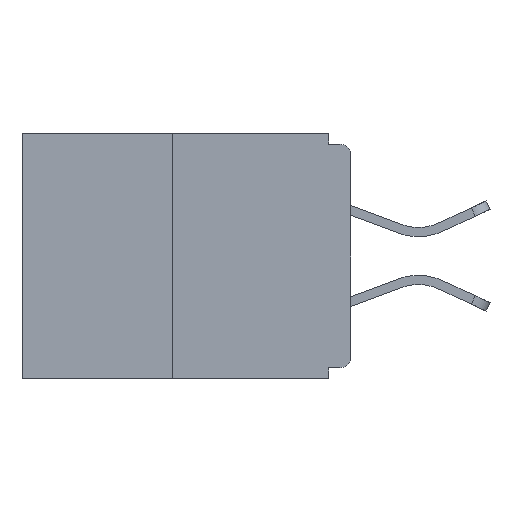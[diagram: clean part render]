
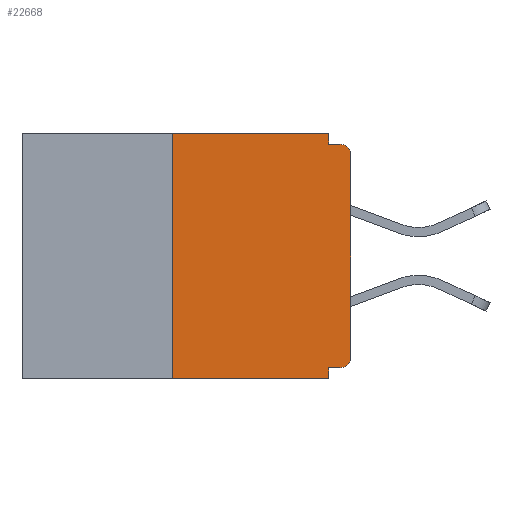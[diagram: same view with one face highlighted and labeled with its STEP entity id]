
A CAD part, left-side view. The second image highlights one B-rep face of the part: STEP entity #22668.
In plain terms, the highlighted planar face has unit normal (-1, 0, 0).
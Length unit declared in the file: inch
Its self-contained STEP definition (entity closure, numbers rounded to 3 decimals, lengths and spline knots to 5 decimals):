
#311 = ORIENTED_EDGE ( 'NONE', *, *, #23160, .F. ) ;
#749 = CARTESIAN_POINT ( 'NONE',  ( 0., 0.46, 0. ) ) ;
#984 = DIRECTION ( 'NONE',  ( -1., 0., 0. ) ) ;
#1036 = VERTEX_POINT ( 'NONE', #2651 ) ;
#1200 = VECTOR ( 'NONE', #20123, 39.37008 ) ;
#1332 = VERTEX_POINT ( 'NONE', #11751 ) ;
#1795 = EDGE_CURVE ( 'NONE', #21712, #1036, #19351, .T. ) ;
#2651 = CARTESIAN_POINT ( 'NONE',  ( 0., 0.015, -0.015 ) ) ;
#2827 = VECTOR ( 'NONE', #16378, 39.37008 ) ;
#3224 = EDGE_LOOP ( 'NONE', ( #311, #25900, #19382, #6486, #30759, #19898, #22731, #23529, #9646, #14262 ) ) ;
#3354 = CARTESIAN_POINT ( 'NONE',  ( 0., 0.25, 0. ) ) ;
#3459 = CARTESIAN_POINT ( 'NONE',  ( 0., 0., 0. ) ) ;
#3608 = CARTESIAN_POINT ( 'NONE',  ( 0., 0.46, -0.343 ) ) ;
#4226 = AXIS2_PLACEMENT_3D ( 'NONE', #27526, #984, #18160 ) ;
#4317 = LINE ( 'NONE', #17866, #1200 ) ;
#6371 = LINE ( 'NONE', #19010, #9063 ) ;
#6486 = ORIENTED_EDGE ( 'NONE', *, *, #20526, .F. ) ;
#7326 = LINE ( 'NONE', #22070, #20362 ) ;
#7821 = VERTEX_POINT ( 'NONE', #9817 ) ;
#8013 = LINE ( 'NONE', #3608, #18004 ) ;
#8146 = DIRECTION ( 'NONE',  ( 1., 0., 0. ) ) ;
#8205 = CARTESIAN_POINT ( 'NONE',  ( 0., 0., -0.328 ) ) ;
#9063 = VECTOR ( 'NONE', #26462, 39.37008 ) ;
#9182 = CARTESIAN_POINT ( 'NONE',  ( 0., 0., -0.313 ) ) ;
#9421 = VERTEX_POINT ( 'NONE', #27793 ) ;
#9646 = ORIENTED_EDGE ( 'NONE', *, *, #12919, .F. ) ;
#9674 = VERTEX_POINT ( 'NONE', #25311 ) ;
#9817 = CARTESIAN_POINT ( 'NONE',  ( 0., 0.015, -0.328 ) ) ;
#10089 = LINE ( 'NONE', #15951, #26540 ) ;
#10485 = LINE ( 'NONE', #3459, #14682 ) ;
#10829 = DIRECTION ( 'NONE',  ( 0., 0., -1. ) ) ;
#11751 = CARTESIAN_POINT ( 'NONE',  ( 0., 0.25, -0.343 ) ) ;
#12376 = AXIS2_PLACEMENT_3D ( 'NONE', #749, #8146, #10829 ) ;
#12567 = VERTEX_POINT ( 'NONE', #3354 ) ;
#12919 = EDGE_CURVE ( 'NONE', #9421, #1036, #7326, .T. ) ;
#14188 = CARTESIAN_POINT ( 'NONE',  ( 0., 0.031, 0. ) ) ;
#14262 = ORIENTED_EDGE ( 'NONE', *, *, #23239, .F. ) ;
#14634 = DIRECTION ( 'NONE',  ( 0., -1., 0. ) ) ;
#14682 = VECTOR ( 'NONE', #22709, 39.37008 ) ;
#15905 = DIRECTION ( 'NONE',  ( 0., -1., 0. ) ) ;
#15951 = CARTESIAN_POINT ( 'NONE',  ( 0., 0.46, 0. ) ) ;
#16243 = CIRCLE ( 'NONE', #28810, 0.015 ) ;
#16259 = VERTEX_POINT ( 'NONE', #31473 ) ;
#16378 = DIRECTION ( 'NONE',  ( 0., 0., -1. ) ) ;
#16776 = EDGE_CURVE ( 'NONE', #7821, #9674, #26425, .T. ) ;
#16782 = CARTESIAN_POINT ( 'NONE',  ( 0., 0., -0.03 ) ) ;
#17866 = CARTESIAN_POINT ( 'NONE',  ( 0., 0.031, -0.343 ) ) ;
#18004 = VECTOR ( 'NONE', #15905, 39.37008 ) ;
#18026 = PLANE ( 'NONE',  #12376 ) ;
#18160 = DIRECTION ( 'NONE',  ( 0., 0., -1. ) ) ;
#19010 = CARTESIAN_POINT ( 'NONE',  ( 0., 0.25, 0. ) ) ;
#19342 = FACE_OUTER_BOUND ( 'NONE', #3224, .T. ) ;
#19351 = CIRCLE ( 'NONE', #4226, 0.015 ) ;
#19382 = ORIENTED_EDGE ( 'NONE', *, *, #25205, .T. ) ;
#19898 = ORIENTED_EDGE ( 'NONE', *, *, #22839, .T. ) ;
#20123 = DIRECTION ( 'NONE',  ( 0., 0., -1. ) ) ;
#20362 = VECTOR ( 'NONE', #14634, 39.37008 ) ;
#20451 = DIRECTION ( 'NONE',  ( 0., 1., 0. ) ) ;
#20526 = EDGE_CURVE ( 'NONE', #9674, #25125, #4317, .T. ) ;
#20714 = VECTOR ( 'NONE', #20451, 39.37008 ) ;
#21712 = VERTEX_POINT ( 'NONE', #16782 ) ;
#22070 = CARTESIAN_POINT ( 'NONE',  ( 0., 0., -0.015 ) ) ;
#22668 = ADVANCED_FACE ( 'NONE', ( #19342 ), #18026, .F. ) ;
#22709 = DIRECTION ( 'NONE',  ( 0., 0., 1. ) ) ;
#22731 = ORIENTED_EDGE ( 'NONE', *, *, #22766, .T. ) ;
#22766 = EDGE_CURVE ( 'NONE', #24740, #21712, #10485, .T. ) ;
#22839 = EDGE_CURVE ( 'NONE', #7821, #24740, #16243, .T. ) ;
#23160 = EDGE_CURVE ( 'NONE', #12567, #16259, #10089, .T. ) ;
#23239 = EDGE_CURVE ( 'NONE', #16259, #9421, #31163, .T. ) ;
#23529 = ORIENTED_EDGE ( 'NONE', *, *, #1795, .T. ) ;
#24740 = VERTEX_POINT ( 'NONE', #9182 ) ;
#25125 = VERTEX_POINT ( 'NONE', #27988 ) ;
#25205 = EDGE_CURVE ( 'NONE', #1332, #25125, #8013, .T. ) ;
#25311 = CARTESIAN_POINT ( 'NONE',  ( 0., 0.031, -0.328 ) ) ;
#25900 = ORIENTED_EDGE ( 'NONE', *, *, #28841, .F. ) ;
#26425 = LINE ( 'NONE', #8205, #20714 ) ;
#26462 = DIRECTION ( 'NONE',  ( 0., 0., 1. ) ) ;
#26540 = VECTOR ( 'NONE', #28881, 39.37008 ) ;
#26862 = CARTESIAN_POINT ( 'NONE',  ( 0., 0.015, -0.313 ) ) ;
#27526 = CARTESIAN_POINT ( 'NONE',  ( 0., 0.015, -0.03 ) ) ;
#27793 = CARTESIAN_POINT ( 'NONE',  ( 0., 0.031, -0.015 ) ) ;
#27988 = CARTESIAN_POINT ( 'NONE',  ( 0., 0.031, -0.343 ) ) ;
#28583 = DIRECTION ( 'NONE',  ( 0., 0., -1. ) ) ;
#28796 = DIRECTION ( 'NONE',  ( -1., 0., 0. ) ) ;
#28810 = AXIS2_PLACEMENT_3D ( 'NONE', #26862, #28796, #28583 ) ;
#28841 = EDGE_CURVE ( 'NONE', #1332, #12567, #6371, .T. ) ;
#28881 = DIRECTION ( 'NONE',  ( 0., -1., 0. ) ) ;
#30759 = ORIENTED_EDGE ( 'NONE', *, *, #16776, .F. ) ;
#31163 = LINE ( 'NONE', #14188, #2827 ) ;
#31473 = CARTESIAN_POINT ( 'NONE',  ( 0., 0.031, 0. ) ) ;
